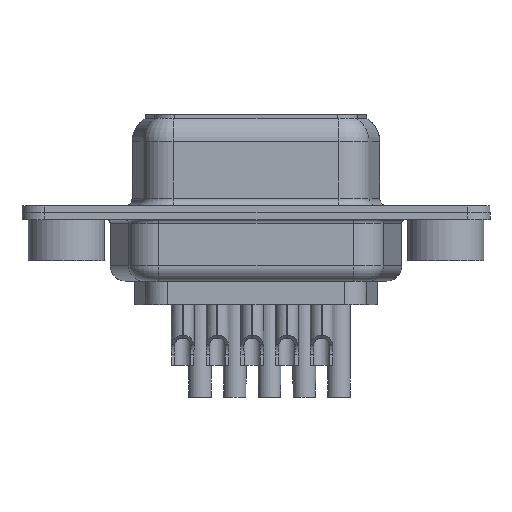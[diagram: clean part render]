
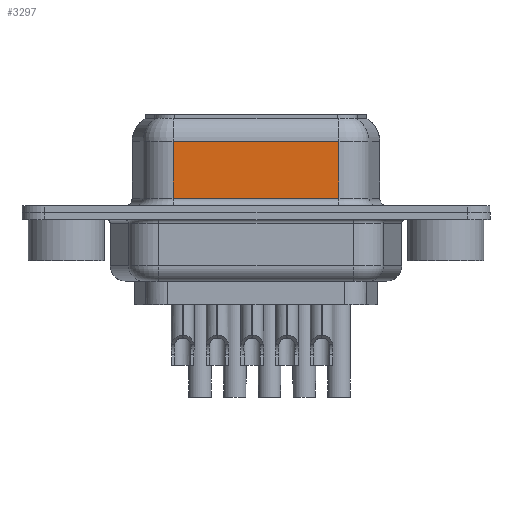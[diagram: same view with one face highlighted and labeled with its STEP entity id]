
A CAD part, front view. The second image highlights one B-rep face of the part: STEP entity #3297.
In plain terms, the highlighted planar face has unit normal (0, -1, 0).
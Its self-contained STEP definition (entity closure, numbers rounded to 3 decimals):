
#1523 = VERTEX_POINT ( 'NONE', #9476 ) ;
#1670 = DIRECTION ( 'NONE',  ( 0., 1., 0. ) ) ;
#2818 = ORIENTED_EDGE ( 'NONE', *, *, #3117, .T. ) ;
#3078 = CARTESIAN_POINT ( 'NONE',  ( 17.957, -3.95, 4.7 ) ) ;
#3117 = EDGE_CURVE ( 'NONE', #1523, #14666, #7841, .T. ) ;
#3297 = ADVANCED_FACE ( 'NONE', ( #9555 ), #10947, .F. ) ;
#3591 = CARTESIAN_POINT ( 'NONE',  ( 17.957, -3.95, 0.95 ) ) ;
#5290 = DIRECTION ( 'NONE',  ( 1., 0., 0. ) ) ;
#6435 = VERTEX_POINT ( 'NONE', #3078 ) ;
#6849 = EDGE_CURVE ( 'NONE', #6435, #8921, #20571, .T. ) ;
#6877 = EDGE_CURVE ( 'NONE', #14666, #8921, #7179, .T. ) ;
#7092 = VECTOR ( 'NONE', #5290, 1000. ) ;
#7179 = LINE ( 'NONE', #18566, #7092 ) ;
#7841 = LINE ( 'NONE', #15474, #18534 ) ;
#8599 = ORIENTED_EDGE ( 'NONE', *, *, #6849, .F. ) ;
#8700 = EDGE_CURVE ( 'NONE', #6435, #1523, #23250, .T. ) ;
#8921 = VERTEX_POINT ( 'NONE', #3591 ) ;
#8980 = AXIS2_PLACEMENT_3D ( 'NONE', #22696, #1670, #16705 ) ;
#9476 = CARTESIAN_POINT ( 'NONE',  ( 7.033, -3.95, 4.7 ) ) ;
#9555 = FACE_OUTER_BOUND ( 'NONE', #10930, .T. ) ;
#10930 = EDGE_LOOP ( 'NONE', ( #8599, #21926, #2818, #21842 ) ) ;
#10947 = PLANE ( 'NONE',  #8980 ) ;
#13861 = VECTOR ( 'NONE', #21285, 1000. ) ;
#14666 = VERTEX_POINT ( 'NONE', #14902 ) ;
#14902 = CARTESIAN_POINT ( 'NONE',  ( 7.033, -3.95, 0.95 ) ) ;
#15108 = VECTOR ( 'NONE', #20210, 1000. ) ;
#15474 = CARTESIAN_POINT ( 'NONE',  ( 7.033, -3.95, 6.45 ) ) ;
#16705 = DIRECTION ( 'NONE',  ( 0., 0., 1. ) ) ;
#18534 = VECTOR ( 'NONE', #23075, 1000. ) ;
#18566 = CARTESIAN_POINT ( 'NONE',  ( 17.957, -3.95, 0.95 ) ) ;
#20210 = DIRECTION ( 'NONE',  ( 0., 0., -1. ) ) ;
#20453 = CARTESIAN_POINT ( 'NONE',  ( 17.957, -3.95, 6.45 ) ) ;
#20571 = LINE ( 'NONE', #20453, #15108 ) ;
#21285 = DIRECTION ( 'NONE',  ( -1., 0., 0. ) ) ;
#21842 = ORIENTED_EDGE ( 'NONE', *, *, #6877, .T. ) ;
#21926 = ORIENTED_EDGE ( 'NONE', *, *, #8700, .T. ) ;
#22696 = CARTESIAN_POINT ( 'NONE',  ( 17.957, -3.95, 6.45 ) ) ;
#23075 = DIRECTION ( 'NONE',  ( 0., 0., -1. ) ) ;
#23250 = LINE ( 'NONE', #23368, #13861 ) ;
#23368 = CARTESIAN_POINT ( 'NONE',  ( 17.957, -3.95, 4.7 ) ) ;
